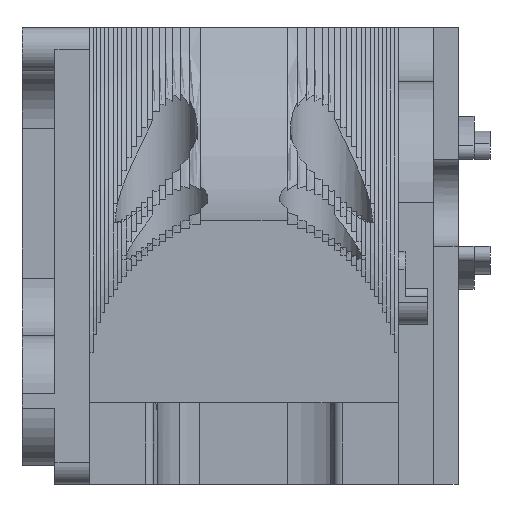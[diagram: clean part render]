
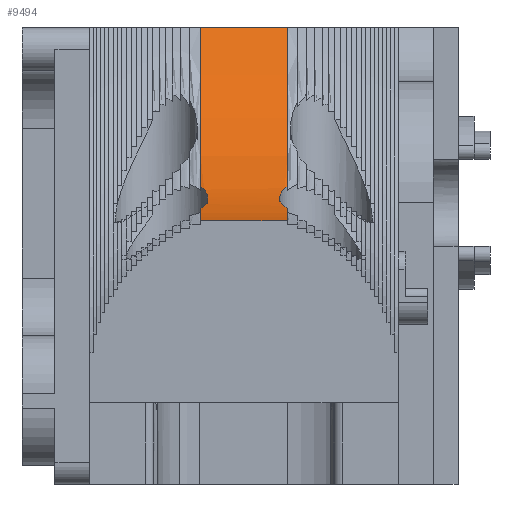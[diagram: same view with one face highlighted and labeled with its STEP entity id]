
A CAD part, left-side view. The second image highlights one B-rep face of the part: STEP entity #9494.
In plain terms, the highlighted cylindrical face has radius 23.607 mm (diameter 47.213 mm), a partial arc.
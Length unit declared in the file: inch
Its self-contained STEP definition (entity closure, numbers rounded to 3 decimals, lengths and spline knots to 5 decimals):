
#421=FACE_OUTER_BOUND('',#929,.T.);
#929=EDGE_LOOP('',(#6637,#6638,#6639,#6640,#6641,#6642,#6643,#6644));
#1408=B_SPLINE_CURVE_WITH_KNOTS('',3,(#14368,#14369,#14370,#14371,#14372,
#14373,#14374,#14375,#14376,#14377),.UNSPECIFIED.,.F.,.F.,(4,2,2,2,4),(-0.67314,
-0.60684,-0.48436,-0.35535,-0.28952),
 .UNSPECIFIED.);
#1425=B_SPLINE_CURVE_WITH_KNOTS('',3,(#14806,#14807,#14808,#14809,#14810,
#14811,#14812,#14813,#14814,#14815),.UNSPECIFIED.,.F.,.F.,(4,2,2,2,4),(0.28952,
0.35535,0.48436,0.60684,0.67314),
 .UNSPECIFIED.);
#1613=LINE('',#14802,#2429);
#1614=LINE('',#14818,#2430);
#2429=VECTOR('',#11610,0.3937);
#2430=VECTOR('',#11615,0.3937);
#3200=CIRCLE('',#10084,0.92939);
#3201=CIRCLE('',#10086,0.92939);
#3229=CIRCLE('',#10145,0.92939);
#3230=CIRCLE('',#10146,0.92939);
#3777=VERTEX_POINT('',#14365);
#3778=VERTEX_POINT('',#14367);
#3827=VERTEX_POINT('',#14620);
#3828=VERTEX_POINT('',#14624);
#3878=VERTEX_POINT('',#14801);
#3879=VERTEX_POINT('',#14803);
#3880=VERTEX_POINT('',#14805);
#3881=VERTEX_POINT('',#14816);
#4787=EDGE_CURVE('',#3778,#3777,#1408,.T.);
#4882=EDGE_CURVE('',#3827,#3778,#3200,.T.);
#4885=EDGE_CURVE('',#3777,#3828,#3201,.T.);
#4964=EDGE_CURVE('',#3828,#3878,#1613,.T.);
#4965=EDGE_CURVE('',#3879,#3878,#3229,.T.);
#4966=EDGE_CURVE('',#3879,#3880,#1425,.T.);
#4967=EDGE_CURVE('',#3881,#3880,#3230,.T.);
#4968=EDGE_CURVE('',#3827,#3881,#1614,.T.);
#6637=ORIENTED_EDGE('',*,*,#4885,.T.);
#6638=ORIENTED_EDGE('',*,*,#4964,.T.);
#6639=ORIENTED_EDGE('',*,*,#4965,.F.);
#6640=ORIENTED_EDGE('',*,*,#4966,.T.);
#6641=ORIENTED_EDGE('',*,*,#4967,.F.);
#6642=ORIENTED_EDGE('',*,*,#4968,.F.);
#6643=ORIENTED_EDGE('',*,*,#4882,.T.);
#6644=ORIENTED_EDGE('',*,*,#4787,.T.);
#9175=CYLINDRICAL_SURFACE('',#10144,0.92939);
#9494=ADVANCED_FACE('',(#421),#9175,.F.);
#10084=AXIS2_PLACEMENT_3D('',#14621,#11441,#11442);
#10086=AXIS2_PLACEMENT_3D('',#14626,#11447,#11448);
#10144=AXIS2_PLACEMENT_3D('',#14800,#11608,#11609);
#10145=AXIS2_PLACEMENT_3D('',#14804,#11611,#11612);
#10146=AXIS2_PLACEMENT_3D('',#14817,#11613,#11614);
#11441=DIRECTION('center_axis',(0.,-1.,0.));
#11442=DIRECTION('ref_axis',(0.,0.,
-1.));
#11447=DIRECTION('center_axis',(0.,-1.,0.));
#11448=DIRECTION('ref_axis',(0.,0.,
-1.));
#11608=DIRECTION('center_axis',(0.,-1.,0.));
#11609=DIRECTION('ref_axis',(0.,0.,
-1.));
#11610=DIRECTION('',(0.,1.,0.));
#11611=DIRECTION('center_axis',(0.,-1.,0.));
#11612=DIRECTION('ref_axis',(1.,0.,0.));
#11613=DIRECTION('center_axis',(0.,-1.,0.));
#11614=DIRECTION('ref_axis',(1.,0.,0.));
#11615=DIRECTION('',(0.,1.,0.));
#14365=CARTESIAN_POINT('',(-1.83919,-0.124,-1.7266));
#14367=CARTESIAN_POINT('',(-1.97521,-0.124,-1.79029));
#14368=CARTESIAN_POINT('Ctrl Pts',(-1.97521,-0.124,
-1.79029));
#14369=CARTESIAN_POINT('Ctrl Pts',(-1.96811,-0.119,
-1.78764));
#14370=CARTESIAN_POINT('Ctrl Pts',(-1.9604,-0.11476,
-1.78466));
#14371=CARTESIAN_POINT('Ctrl Pts',(-1.9376,-0.10531,
-1.77547));
#14372=CARTESIAN_POINT('Ctrl Pts',(-1.92177,-0.10245,
-1.76859));
#14373=CARTESIAN_POINT('Ctrl Pts',(-1.89185,-0.10245,
-1.75465));
#14374=CARTESIAN_POINT('Ctrl Pts',(-1.87565,-0.1056,
-1.74653));
#14375=CARTESIAN_POINT('Ctrl Pts',(-1.85317,-0.11521,
-1.73447));
#14376=CARTESIAN_POINT('Ctrl Pts',(-1.8459,-0.11927,
-1.73044));
#14377=CARTESIAN_POINT('Ctrl Pts',(-1.83919,-0.124,
-1.7266));
#14620=CARTESIAN_POINT('',(-2.1,-0.124,-1.82711));
#14621=CARTESIAN_POINT('Origin',(-2.3,-0.124,-0.9195));
#14624=CARTESIAN_POINT('',(-1.43903,-0.124,-1.2695));
#14626=CARTESIAN_POINT('Origin',(-2.3,-0.124,-0.9195));
#14800=CARTESIAN_POINT('Origin',(-2.3,-0.2965,-0.9195));
#14801=CARTESIAN_POINT('',(-1.43903,0.126,-1.2695));
#14802=CARTESIAN_POINT('',(-1.43903,-0.2965,-1.2695));
#14803=CARTESIAN_POINT('',(-1.83919,0.126,-1.7266));
#14804=CARTESIAN_POINT('Origin',(-2.3,0.126,-0.9195));
#14805=CARTESIAN_POINT('',(-1.97521,0.126,-1.79029));
#14806=CARTESIAN_POINT('Ctrl Pts',(-1.83919,0.126,
-1.7266));
#14807=CARTESIAN_POINT('Ctrl Pts',(-1.8459,0.12127,
-1.73044));
#14808=CARTESIAN_POINT('Ctrl Pts',(-1.85317,0.11721,
-1.73447));
#14809=CARTESIAN_POINT('Ctrl Pts',(-1.87565,0.1076,
-1.74653));
#14810=CARTESIAN_POINT('Ctrl Pts',(-1.89185,0.10445,
-1.75465));
#14811=CARTESIAN_POINT('Ctrl Pts',(-1.92177,0.10445,
-1.76859));
#14812=CARTESIAN_POINT('Ctrl Pts',(-1.9376,0.10731,
-1.77547));
#14813=CARTESIAN_POINT('Ctrl Pts',(-1.9604,0.11676,
-1.78466));
#14814=CARTESIAN_POINT('Ctrl Pts',(-1.96811,0.121,
-1.78764));
#14815=CARTESIAN_POINT('Ctrl Pts',(-1.97521,0.126,
-1.79029));
#14816=CARTESIAN_POINT('',(-2.1,0.126,-1.82711));
#14817=CARTESIAN_POINT('Origin',(-2.3,0.126,-0.9195));
#14818=CARTESIAN_POINT('',(-2.1,-0.2965,-1.82711));
